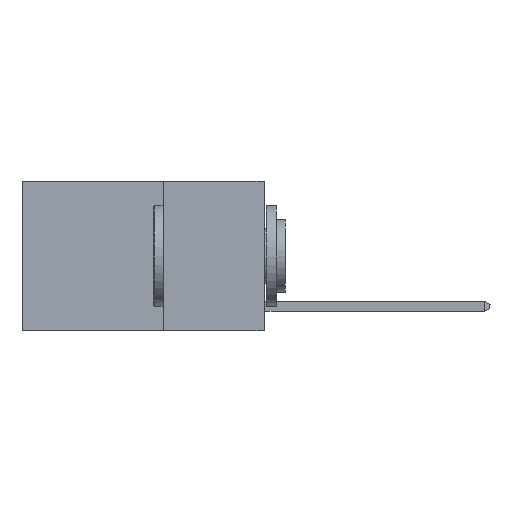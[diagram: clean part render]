
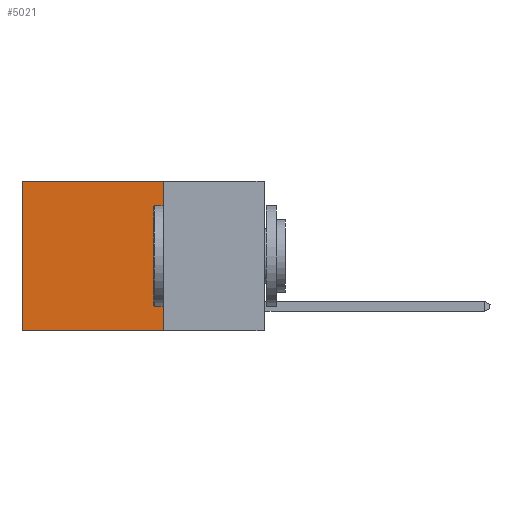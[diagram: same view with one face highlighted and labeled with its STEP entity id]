
A CAD part, left-side view. The second image highlights one B-rep face of the part: STEP entity #5021.
In plain terms, the highlighted planar face has unit normal (-1, 0, 0).
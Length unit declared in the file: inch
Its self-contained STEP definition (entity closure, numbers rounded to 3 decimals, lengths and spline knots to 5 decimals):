
#421 = VECTOR ( 'NONE', #7235, 39.37008 ) ;
#1715 = PLANE ( 'NONE',  #20647 ) ;
#3126 = VERTEX_POINT ( 'NONE', #22354 ) ;
#3829 = VECTOR ( 'NONE', #25804, 39.37008 ) ;
#4403 = LINE ( 'NONE', #16707, #421 ) ;
#5021 = ADVANCED_FACE ( 'NONE', ( #18607 ), #1715, .F. ) ;
#5626 = ORIENTED_EDGE ( 'NONE', *, *, #23473, .F. ) ;
#7058 = EDGE_LOOP ( 'NONE', ( #12448, #5626, #14982, #18921 ) ) ;
#7235 = DIRECTION ( 'NONE',  ( 0., 1., 0. ) ) ;
#8400 = DIRECTION ( 'NONE',  ( 1., 0., 0. ) ) ;
#8571 = EDGE_CURVE ( 'NONE', #12734, #23680, #23676, .T. ) ;
#9963 = LINE ( 'NONE', #23230, #3829 ) ;
#10727 = DIRECTION ( 'NONE',  ( 0., 0., -1. ) ) ;
#11543 = CARTESIAN_POINT ( 'NONE',  ( 0.2625, 0.25, 0. ) ) ;
#12448 = ORIENTED_EDGE ( 'NONE', *, *, #28999, .T. ) ;
#12734 = VERTEX_POINT ( 'NONE', #11543 ) ;
#14046 = CARTESIAN_POINT ( 'NONE',  ( 0.2625, 0.6, 0. ) ) ;
#14817 = CARTESIAN_POINT ( 'NONE',  ( 0.2625, 0.25, 0. ) ) ;
#14982 = ORIENTED_EDGE ( 'NONE', *, *, #27369, .F. ) ;
#16707 = CARTESIAN_POINT ( 'NONE',  ( 0.2625, 0.25, -0.37 ) ) ;
#17240 = VECTOR ( 'NONE', #28753, 39.37008 ) ;
#17478 = VECTOR ( 'NONE', #23845, 39.37008 ) ;
#18607 = FACE_OUTER_BOUND ( 'NONE', #7058, .T. ) ;
#18921 = ORIENTED_EDGE ( 'NONE', *, *, #8571, .T. ) ;
#20647 = AXIS2_PLACEMENT_3D ( 'NONE', #29385, #8400, #10727 ) ;
#21698 = CARTESIAN_POINT ( 'NONE',  ( 0.2625, 0.6, 0. ) ) ;
#22354 = CARTESIAN_POINT ( 'NONE',  ( 0.2625, 0.6, -0.37 ) ) ;
#23230 = CARTESIAN_POINT ( 'NONE',  ( 0.2625, 0.25, 0. ) ) ;
#23473 = EDGE_CURVE ( 'NONE', #29208, #3126, #4403, .T. ) ;
#23676 = LINE ( 'NONE', #14817, #17478 ) ;
#23680 = VERTEX_POINT ( 'NONE', #21698 ) ;
#23845 = DIRECTION ( 'NONE',  ( 0., 1., 0. ) ) ;
#25804 = DIRECTION ( 'NONE',  ( 0., 0., -1. ) ) ;
#26242 = CARTESIAN_POINT ( 'NONE',  ( 0.2625, 0.25, -0.37 ) ) ;
#27114 = LINE ( 'NONE', #14046, #17240 ) ;
#27369 = EDGE_CURVE ( 'NONE', #12734, #29208, #9963, .T. ) ;
#28753 = DIRECTION ( 'NONE',  ( 0., 0., -1. ) ) ;
#28999 = EDGE_CURVE ( 'NONE', #23680, #3126, #27114, .T. ) ;
#29208 = VERTEX_POINT ( 'NONE', #26242 ) ;
#29385 = CARTESIAN_POINT ( 'NONE',  ( 0.2625, 0.25, 0. ) ) ;
